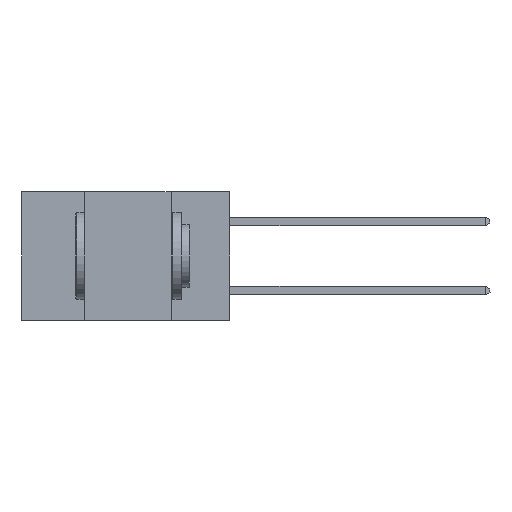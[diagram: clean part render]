
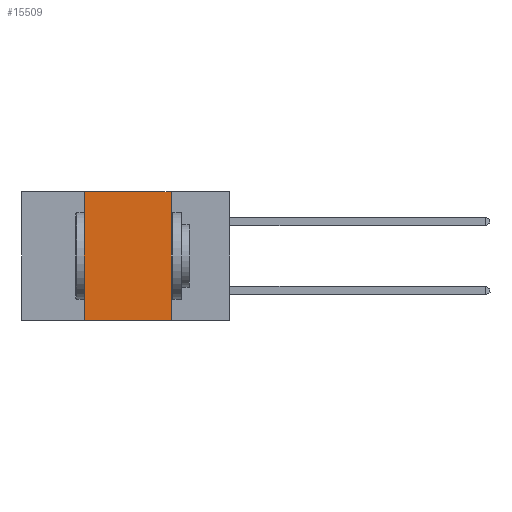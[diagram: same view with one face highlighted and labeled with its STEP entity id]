
A CAD part, left-side view. The second image highlights one B-rep face of the part: STEP entity #15509.
In plain terms, the highlighted planar face has unit normal (-1, 0, 0).
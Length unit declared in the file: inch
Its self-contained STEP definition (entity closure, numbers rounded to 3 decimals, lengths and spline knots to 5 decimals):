
#897 = VERTEX_POINT ( 'NONE', #25705 ) ;
#1815 = FACE_OUTER_BOUND ( 'NONE', #9732, .T. ) ;
#2555 = AXIS2_PLACEMENT_3D ( 'NONE', #6634, #4345, #21717 ) ;
#2646 = EDGE_CURVE ( 'NONE', #10403, #23772, #8142, .T. ) ;
#3862 = DIRECTION ( 'NONE',  ( 0., -1., 0. ) ) ;
#4341 = CARTESIAN_POINT ( 'NONE',  ( 0., 0.17, 0. ) ) ;
#4345 = DIRECTION ( 'NONE',  ( 1., 0., 0. ) ) ;
#5906 = EDGE_CURVE ( 'NONE', #25218, #897, #9669, .T. ) ;
#6617 = CARTESIAN_POINT ( 'NONE',  ( 0., 0.42, 0. ) ) ;
#6634 = CARTESIAN_POINT ( 'NONE',  ( 0., 0.6, 0. ) ) ;
#7094 = EDGE_CURVE ( 'NONE', #10403, #897, #27541, .T. ) ;
#8142 = LINE ( 'NONE', #17415, #20967 ) ;
#9176 = CARTESIAN_POINT ( 'NONE',  ( 0., 0.42, -0.37 ) ) ;
#9669 = LINE ( 'NONE', #15926, #20495 ) ;
#9732 = EDGE_LOOP ( 'NONE', ( #18404, #10764, #22715, #26586 ) ) ;
#10264 = VECTOR ( 'NONE', #17155, 39.37008 ) ;
#10403 = VERTEX_POINT ( 'NONE', #9176 ) ;
#10764 = ORIENTED_EDGE ( 'NONE', *, *, #16545, .F. ) ;
#11565 = PLANE ( 'NONE',  #2555 ) ;
#15509 = ADVANCED_FACE ( 'NONE', ( #1815 ), #11565, .F. ) ;
#15926 = CARTESIAN_POINT ( 'NONE',  ( 0., 0.17, 0. ) ) ;
#16343 = VECTOR ( 'NONE', #3862, 39.37008 ) ;
#16545 = EDGE_CURVE ( 'NONE', #23772, #25218, #23404, .T. ) ;
#16816 = CARTESIAN_POINT ( 'NONE',  ( 0., 0.6, 0. ) ) ;
#17155 = DIRECTION ( 'NONE',  ( 0., -1., 0. ) ) ;
#17415 = CARTESIAN_POINT ( 'NONE',  ( 0., 0.42, 0. ) ) ;
#17887 = DIRECTION ( 'NONE',  ( 0., 0., -1. ) ) ;
#18404 = ORIENTED_EDGE ( 'NONE', *, *, #5906, .F. ) ;
#20495 = VECTOR ( 'NONE', #17887, 39.37008 ) ;
#20967 = VECTOR ( 'NONE', #24599, 39.37008 ) ;
#21089 = CARTESIAN_POINT ( 'NONE',  ( 0., 0.6, -0.37 ) ) ;
#21717 = DIRECTION ( 'NONE',  ( 0., 0., -1. ) ) ;
#22715 = ORIENTED_EDGE ( 'NONE', *, *, #2646, .F. ) ;
#23404 = LINE ( 'NONE', #16816, #16343 ) ;
#23772 = VERTEX_POINT ( 'NONE', #6617 ) ;
#24599 = DIRECTION ( 'NONE',  ( 0., 0., 1. ) ) ;
#25218 = VERTEX_POINT ( 'NONE', #4341 ) ;
#25705 = CARTESIAN_POINT ( 'NONE',  ( 0., 0.17, -0.37 ) ) ;
#26586 = ORIENTED_EDGE ( 'NONE', *, *, #7094, .T. ) ;
#27541 = LINE ( 'NONE', #21089, #10264 ) ;
